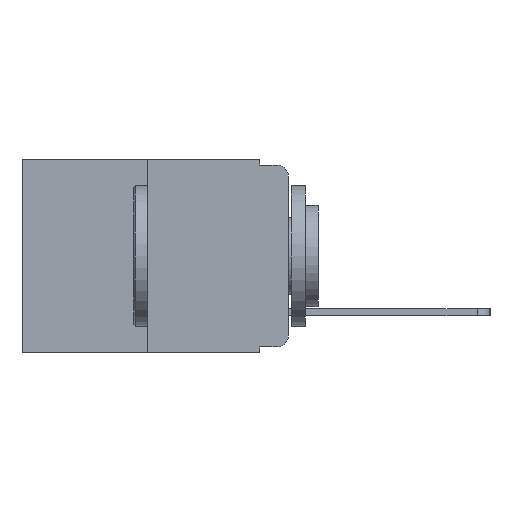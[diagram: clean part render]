
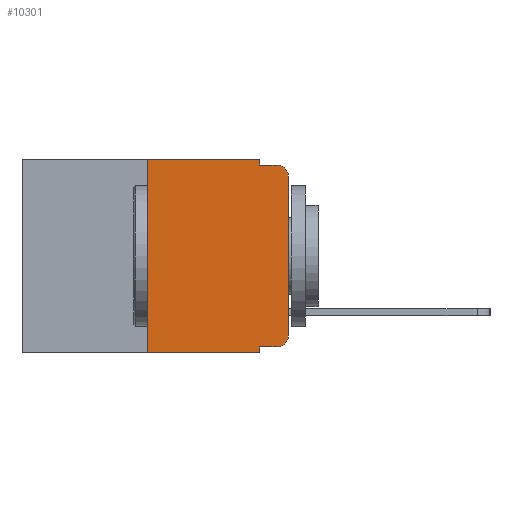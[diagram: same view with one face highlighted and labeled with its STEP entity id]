
A CAD part, left-side view. The second image highlights one B-rep face of the part: STEP entity #10301.
In plain terms, the highlighted planar face has unit normal (-1, 0, 0).
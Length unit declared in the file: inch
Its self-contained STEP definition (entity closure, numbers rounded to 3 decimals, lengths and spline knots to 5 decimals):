
#38 = VECTOR ( 'NONE', #9374, 39.37008 ) ;
#248 = CARTESIAN_POINT ( 'NONE',  ( 0., 0., 0. ) ) ;
#266 = ORIENTED_EDGE ( 'NONE', *, *, #1765, .F. ) ;
#352 = VERTEX_POINT ( 'NONE', #9877 ) ;
#444 = ORIENTED_EDGE ( 'NONE', *, *, #1528, .F. ) ;
#653 = DIRECTION ( 'NONE',  ( -1., 0., 0. ) ) ;
#697 = DIRECTION ( 'NONE',  ( 0., 0., -1. ) ) ;
#747 = LINE ( 'NONE', #248, #3062 ) ;
#1108 = EDGE_CURVE ( 'NONE', #7388, #7095, #11059, .T. ) ;
#1222 = AXIS2_PLACEMENT_3D ( 'NONE', #12111, #6594, #697 ) ;
#1229 = ORIENTED_EDGE ( 'NONE', *, *, #1851, .T. ) ;
#1352 = ORIENTED_EDGE ( 'NONE', *, *, #6391, .F. ) ;
#1528 = EDGE_CURVE ( 'NONE', #3094, #352, #8165, .T. ) ;
#1765 = EDGE_CURVE ( 'NONE', #7388, #5975, #6083, .T. ) ;
#1839 = ORIENTED_EDGE ( 'NONE', *, *, #6152, .T. ) ;
#1851 = EDGE_CURVE ( 'NONE', #6103, #5975, #8014, .T. ) ;
#2265 = CARTESIAN_POINT ( 'NONE',  ( 0., 0.051, 0. ) ) ;
#2683 = LINE ( 'NONE', #8440, #38 ) ;
#2902 = DIRECTION ( 'NONE',  ( 0., 0., -1. ) ) ;
#2999 = DIRECTION ( 'NONE',  ( 0., -1., 0. ) ) ;
#3001 = VECTOR ( 'NONE', #2999, 39.37008 ) ;
#3025 = CARTESIAN_POINT ( 'NONE',  ( 0., 0.051, 0. ) ) ;
#3062 = VECTOR ( 'NONE', #8088, 39.37008 ) ;
#3094 = VERTEX_POINT ( 'NONE', #4749 ) ;
#3223 = CARTESIAN_POINT ( 'NONE',  ( 0., 0.051, 0. ) ) ;
#3300 = DIRECTION ( 'NONE',  ( 0., 0., -1. ) ) ;
#3353 = DIRECTION ( 'NONE',  ( 1., 0., 0. ) ) ;
#3453 = CARTESIAN_POINT ( 'NONE',  ( 0., 0.051, -0.333 ) ) ;
#3498 = VECTOR ( 'NONE', #2902, 39.37008 ) ;
#3547 = EDGE_CURVE ( 'NONE', #7941, #352, #7858, .T. ) ;
#3588 = CIRCLE ( 'NONE', #7705, 0.02 ) ;
#3624 = CARTESIAN_POINT ( 'NONE',  ( 0., 0.25, 0. ) ) ;
#4149 = CARTESIAN_POINT ( 'NONE',  ( 0., 0., -0.313 ) ) ;
#4412 = VERTEX_POINT ( 'NONE', #11625 ) ;
#4482 = ORIENTED_EDGE ( 'NONE', *, *, #3547, .T. ) ;
#4710 = CARTESIAN_POINT ( 'NONE',  ( 0., 0.051, -0.333 ) ) ;
#4749 = CARTESIAN_POINT ( 'NONE',  ( 0., 0.051, -0.01 ) ) ;
#4813 = CARTESIAN_POINT ( 'NONE',  ( 0., 0.473, -0.343 ) ) ;
#4876 = AXIS2_PLACEMENT_3D ( 'NONE', #9105, #3353, #10016 ) ;
#5085 = VERTEX_POINT ( 'NONE', #3223 ) ;
#5462 = VECTOR ( 'NONE', #7142, 39.37008 ) ;
#5975 = VERTEX_POINT ( 'NONE', #10595 ) ;
#6083 = LINE ( 'NONE', #3025, #3498 ) ;
#6103 = VERTEX_POINT ( 'NONE', #10750 ) ;
#6152 = EDGE_CURVE ( 'NONE', #8947, #7941, #747, .T. ) ;
#6391 = EDGE_CURVE ( 'NONE', #6103, #4412, #10521, .T. ) ;
#6454 = DIRECTION ( 'NONE',  ( 0., -1., 0. ) ) ;
#6554 = CARTESIAN_POINT ( 'NONE',  ( 0., 0.02, -0.313 ) ) ;
#6594 = DIRECTION ( 'NONE',  ( -1., 0., 0. ) ) ;
#7095 = VERTEX_POINT ( 'NONE', #11590 ) ;
#7142 = DIRECTION ( 'NONE',  ( 0., -1., 0. ) ) ;
#7225 = PLANE ( 'NONE',  #4876 ) ;
#7388 = VERTEX_POINT ( 'NONE', #4710 ) ;
#7518 = DIRECTION ( 'NONE',  ( 0., 0., -1. ) ) ;
#7521 = ORIENTED_EDGE ( 'NONE', *, *, #10765, .F. ) ;
#7705 = AXIS2_PLACEMENT_3D ( 'NONE', #6554, #653, #7518 ) ;
#7814 = ORIENTED_EDGE ( 'NONE', *, *, #1108, .T. ) ;
#7858 = CIRCLE ( 'NONE', #1222, 0.02 ) ;
#7902 = EDGE_CURVE ( 'NONE', #7095, #8947, #3588, .T. ) ;
#7941 = VERTEX_POINT ( 'NONE', #11215 ) ;
#8014 = LINE ( 'NONE', #4813, #5462 ) ;
#8088 = DIRECTION ( 'NONE',  ( 0., 0., 1. ) ) ;
#8165 = LINE ( 'NONE', #11850, #3001 ) ;
#8440 = CARTESIAN_POINT ( 'NONE',  ( 0., 0.473, 0. ) ) ;
#8607 = VECTOR ( 'NONE', #6454, 39.37008 ) ;
#8762 = EDGE_LOOP ( 'NONE', ( #1839, #4482, #444, #7521, #10845, #1352, #1229, #266, #7814, #9122 ) ) ;
#8947 = VERTEX_POINT ( 'NONE', #4149 ) ;
#9059 = FACE_OUTER_BOUND ( 'NONE', #8762, .T. ) ;
#9105 = CARTESIAN_POINT ( 'NONE',  ( 0., 0.473, 0. ) ) ;
#9122 = ORIENTED_EDGE ( 'NONE', *, *, #7902, .T. ) ;
#9374 = DIRECTION ( 'NONE',  ( 0., -1., 0. ) ) ;
#9877 = CARTESIAN_POINT ( 'NONE',  ( 0., 0.02, -0.01 ) ) ;
#10016 = DIRECTION ( 'NONE',  ( 0., 0., -1. ) ) ;
#10274 = DIRECTION ( 'NONE',  ( 0., 0., 1. ) ) ;
#10301 = ADVANCED_FACE ( 'NONE', ( #9059 ), #7225, .F. ) ;
#10521 = LINE ( 'NONE', #3624, #10805 ) ;
#10595 = CARTESIAN_POINT ( 'NONE',  ( 0., 0.051, -0.343 ) ) ;
#10750 = CARTESIAN_POINT ( 'NONE',  ( 0., 0.25, -0.343 ) ) ;
#10765 = EDGE_CURVE ( 'NONE', #5085, #3094, #11195, .T. ) ;
#10805 = VECTOR ( 'NONE', #10274, 39.37008 ) ;
#10845 = ORIENTED_EDGE ( 'NONE', *, *, #11244, .F. ) ;
#10914 = VECTOR ( 'NONE', #3300, 39.37008 ) ;
#11059 = LINE ( 'NONE', #3453, #8607 ) ;
#11195 = LINE ( 'NONE', #2265, #10914 ) ;
#11215 = CARTESIAN_POINT ( 'NONE',  ( 0., 0., -0.03 ) ) ;
#11244 = EDGE_CURVE ( 'NONE', #4412, #5085, #2683, .T. ) ;
#11590 = CARTESIAN_POINT ( 'NONE',  ( 0., 0.02, -0.333 ) ) ;
#11625 = CARTESIAN_POINT ( 'NONE',  ( 0., 0.25, 0. ) ) ;
#11850 = CARTESIAN_POINT ( 'NONE',  ( 0., 0.051, -0.01 ) ) ;
#12111 = CARTESIAN_POINT ( 'NONE',  ( 0., 0.02, -0.03 ) ) ;
